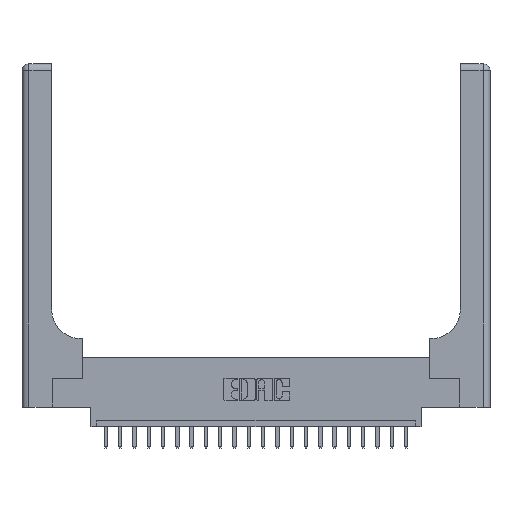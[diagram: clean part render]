
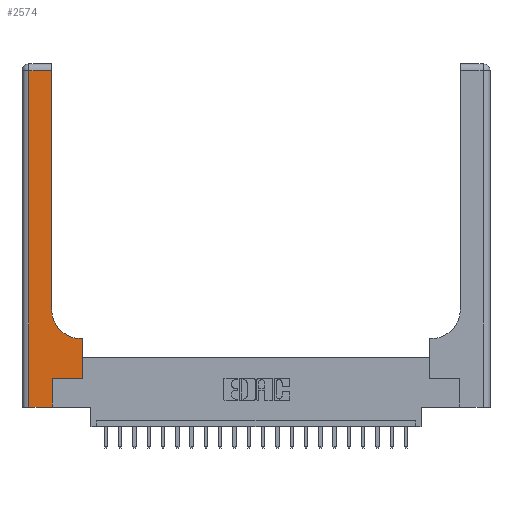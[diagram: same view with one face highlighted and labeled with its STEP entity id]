
A CAD part, top view. The second image highlights one B-rep face of the part: STEP entity #2574.
In plain terms, the highlighted planar face has unit normal (0, 0, 1).
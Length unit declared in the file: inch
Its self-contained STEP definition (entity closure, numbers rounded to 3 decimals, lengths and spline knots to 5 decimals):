
#70 = CARTESIAN_POINT ( 'NONE',  ( 0.06, 2.94, 0.37 ) ) ;
#177 = AXIS2_PLACEMENT_3D ( 'NONE', #15637, #3872, #19307 ) ;
#265 = ORIENTED_EDGE ( 'NONE', *, *, #324, .T. ) ;
#298 = VERTEX_POINT ( 'NONE', #18319 ) ;
#324 = EDGE_CURVE ( 'NONE', #17846, #4357, #1480, .T. ) ;
#437 = CARTESIAN_POINT ( 'NONE',  ( 0., 2.94, 0.37 ) ) ;
#514 = VECTOR ( 'NONE', #13669, 39.37008 ) ;
#563 = DIRECTION ( 'NONE',  ( -1., 0., 0. ) ) ;
#739 = EDGE_CURVE ( 'NONE', #7945, #14595, #14889, .T. ) ;
#909 = CARTESIAN_POINT ( 'NONE',  ( 0.26, 3., 0.37 ) ) ;
#1071 = VERTEX_POINT ( 'NONE', #70 ) ;
#1435 = DIRECTION ( 'NONE',  ( 0., -1., 0. ) ) ;
#1480 = LINE ( 'NONE', #8155, #6758 ) ;
#1552 = LINE ( 'NONE', #437, #514 ) ;
#1970 = CIRCLE ( 'NONE', #177, 0.25 ) ;
#2135 = CARTESIAN_POINT ( 'NONE',  ( 0.06, 0., 0.37 ) ) ;
#2458 = CARTESIAN_POINT ( 'NONE',  ( 0.26, 0.85, 0.37 ) ) ;
#2469 = LINE ( 'NONE', #909, #12178 ) ;
#2574 = ADVANCED_FACE ( 'NONE', ( #13742 ), #11386, .F. ) ;
#2683 = CARTESIAN_POINT ( 'NONE',  ( 0.26, 2.94, 0.37 ) ) ;
#2923 = EDGE_CURVE ( 'NONE', #11772, #3480, #2469, .T. ) ;
#3076 = CARTESIAN_POINT ( 'NONE',  ( 0., 3., 0.37 ) ) ;
#3094 = DIRECTION ( 'NONE',  ( -1., 0., 0. ) ) ;
#3236 = CARTESIAN_POINT ( 'NONE',  ( 0.265, 0.25, 0.37 ) ) ;
#3398 = CARTESIAN_POINT ( 'NONE',  ( 0.265, 0., 0.37 ) ) ;
#3480 = VERTEX_POINT ( 'NONE', #2683 ) ;
#3573 = VECTOR ( 'NONE', #3094, 39.37008 ) ;
#3858 = DIRECTION ( 'NONE',  ( 0., 0., -1. ) ) ;
#3862 = CARTESIAN_POINT ( 'NONE',  ( 0.528, 0.25, 0.37 ) ) ;
#3872 = DIRECTION ( 'NONE',  ( 0., 0., -1. ) ) ;
#4024 = AXIS2_PLACEMENT_3D ( 'NONE', #3076, #3858, #563 ) ;
#4357 = VERTEX_POINT ( 'NONE', #5213 ) ;
#4707 = DIRECTION ( 'NONE',  ( 1., 0., 0. ) ) ;
#4845 = ORIENTED_EDGE ( 'NONE', *, *, #739, .T. ) ;
#5062 = ORIENTED_EDGE ( 'NONE', *, *, #14896, .T. ) ;
#5213 = CARTESIAN_POINT ( 'NONE',  ( 0.265, 0., 0.37 ) ) ;
#5808 = VECTOR ( 'NONE', #21330, 39.37008 ) ;
#5967 = ORIENTED_EDGE ( 'NONE', *, *, #12487, .T. ) ;
#6256 = EDGE_LOOP ( 'NONE', ( #18429, #19083, #15234, #265, #5062, #5967, #13302, #4845, #10366 ) ) ;
#6474 = CARTESIAN_POINT ( 'NONE',  ( 0.265, 0.25, 0.37 ) ) ;
#6758 = VECTOR ( 'NONE', #4707, 39.37008 ) ;
#6818 = LINE ( 'NONE', #7989, #11244 ) ;
#7400 = CARTESIAN_POINT ( 'NONE',  ( 0.51, 0.6, 0.37 ) ) ;
#7766 = VECTOR ( 'NONE', #9687, 39.37008 ) ;
#7945 = VERTEX_POINT ( 'NONE', #17654 ) ;
#7989 = CARTESIAN_POINT ( 'NONE',  ( 0.06, 3., 0.37 ) ) ;
#8155 = CARTESIAN_POINT ( 'NONE',  ( 0., 0., 0.37 ) ) ;
#9162 = DIRECTION ( 'NONE',  ( 0., 1., 0. ) ) ;
#9687 = DIRECTION ( 'NONE',  ( 1., 0., 0. ) ) ;
#10000 = CARTESIAN_POINT ( 'NONE',  ( 0.26, 0.6, 0.37 ) ) ;
#10366 = ORIENTED_EDGE ( 'NONE', *, *, #12815, .T. ) ;
#11244 = VECTOR ( 'NONE', #1435, 39.37008 ) ;
#11386 = PLANE ( 'NONE',  #4024 ) ;
#11772 = VERTEX_POINT ( 'NONE', #2458 ) ;
#12178 = VECTOR ( 'NONE', #21175, 39.37008 ) ;
#12487 = EDGE_CURVE ( 'NONE', #19480, #298, #17995, .T. ) ;
#12815 = EDGE_CURVE ( 'NONE', #14595, #11772, #1970, .T. ) ;
#13038 = LINE ( 'NONE', #3862, #18322 ) ;
#13302 = ORIENTED_EDGE ( 'NONE', *, *, #20782, .T. ) ;
#13669 = DIRECTION ( 'NONE',  ( -1., 0., 0. ) ) ;
#13742 = FACE_OUTER_BOUND ( 'NONE', #6256, .T. ) ;
#14595 = VERTEX_POINT ( 'NONE', #7400 ) ;
#14889 = LINE ( 'NONE', #10000, #3573 ) ;
#14896 = EDGE_CURVE ( 'NONE', #4357, #19480, #19211, .T. ) ;
#15234 = ORIENTED_EDGE ( 'NONE', *, *, #16937, .T. ) ;
#15637 = CARTESIAN_POINT ( 'NONE',  ( 0.51, 0.85, 0.37 ) ) ;
#15708 = EDGE_CURVE ( 'NONE', #3480, #1071, #1552, .T. ) ;
#16937 = EDGE_CURVE ( 'NONE', #1071, #17846, #6818, .T. ) ;
#17654 = CARTESIAN_POINT ( 'NONE',  ( 0.528, 0.6, 0.37 ) ) ;
#17846 = VERTEX_POINT ( 'NONE', #2135 ) ;
#17995 = LINE ( 'NONE', #6474, #7766 ) ;
#18319 = CARTESIAN_POINT ( 'NONE',  ( 0.528, 0.25, 0.37 ) ) ;
#18322 = VECTOR ( 'NONE', #9162, 39.37008 ) ;
#18429 = ORIENTED_EDGE ( 'NONE', *, *, #2923, .T. ) ;
#19083 = ORIENTED_EDGE ( 'NONE', *, *, #15708, .T. ) ;
#19211 = LINE ( 'NONE', #3398, #5808 ) ;
#19307 = DIRECTION ( 'NONE',  ( 1., 0., 0. ) ) ;
#19480 = VERTEX_POINT ( 'NONE', #3236 ) ;
#20782 = EDGE_CURVE ( 'NONE', #298, #7945, #13038, .T. ) ;
#21175 = DIRECTION ( 'NONE',  ( 0., 1., 0. ) ) ;
#21330 = DIRECTION ( 'NONE',  ( 0., 1., 0. ) ) ;
